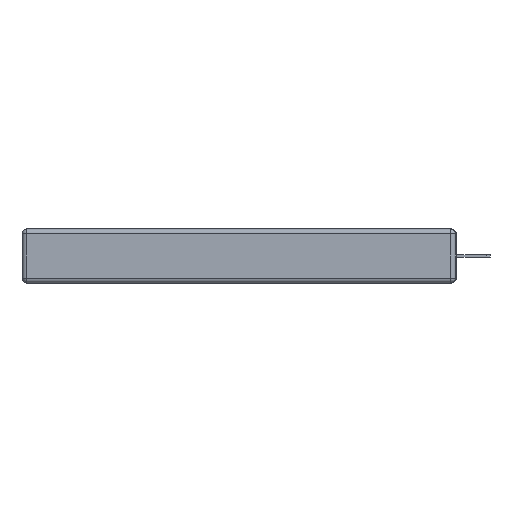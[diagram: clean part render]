
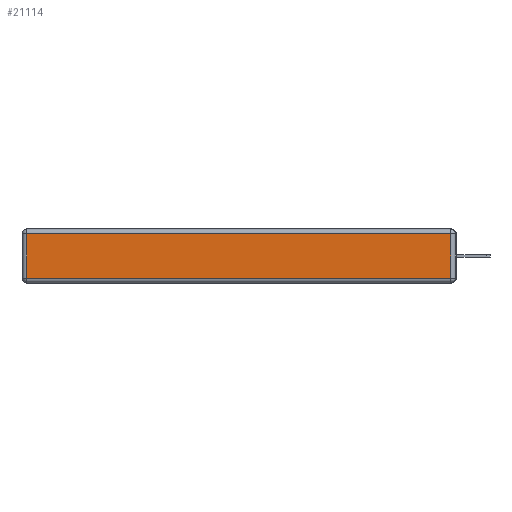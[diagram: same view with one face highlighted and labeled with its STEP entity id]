
A CAD part, left-side view. The second image highlights one B-rep face of the part: STEP entity #21114.
In plain terms, the highlighted planar face has unit normal (-1, 0, 0).
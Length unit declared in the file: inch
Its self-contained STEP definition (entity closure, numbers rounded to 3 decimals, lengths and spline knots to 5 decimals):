
#249 = ORIENTED_EDGE ( 'NONE', *, *, #13192, .T. ) ;
#598 = CARTESIAN_POINT ( 'NONE',  ( 0., 0.03, -0.03 ) ) ;
#813 = VERTEX_POINT ( 'NONE', #15859 ) ;
#1309 = DIRECTION ( 'NONE',  ( 0., 0., 1. ) ) ;
#1898 = ORIENTED_EDGE ( 'NONE', *, *, #19067, .T. ) ;
#2978 = CARTESIAN_POINT ( 'NONE',  ( 0., 0., -0.343 ) ) ;
#3934 = EDGE_LOOP ( 'NONE', ( #6004, #249, #11787, #1898 ) ) ;
#4666 = VECTOR ( 'NONE', #4872, 39.37008 ) ;
#4684 = DIRECTION ( 'NONE',  ( 0., 0., -1. ) ) ;
#4872 = DIRECTION ( 'NONE',  ( 0., 0., 1. ) ) ;
#5842 = VERTEX_POINT ( 'NONE', #19207 ) ;
#6004 = ORIENTED_EDGE ( 'NONE', *, *, #18140, .T. ) ;
#6305 = PLANE ( 'NONE',  #6589 ) ;
#6589 = AXIS2_PLACEMENT_3D ( 'NONE', #2978, #16469, #1309 ) ;
#7566 = CARTESIAN_POINT ( 'NONE',  ( 0., 0., -0.313 ) ) ;
#10645 = DIRECTION ( 'NONE',  ( 0., -1., 0. ) ) ;
#10928 = EDGE_CURVE ( 'NONE', #14163, #813, #13548, .T. ) ;
#11065 = VERTEX_POINT ( 'NONE', #17620 ) ;
#11787 = ORIENTED_EDGE ( 'NONE', *, *, #10928, .T. ) ;
#12101 = CARTESIAN_POINT ( 'NONE',  ( 0., 2.75, -0.03 ) ) ;
#13192 = EDGE_CURVE ( 'NONE', #11065, #14163, #13281, .T. ) ;
#13281 = LINE ( 'NONE', #20012, #4666 ) ;
#13548 = LINE ( 'NONE', #12101, #15796 ) ;
#14099 = LINE ( 'NONE', #7566, #18890 ) ;
#14163 = VERTEX_POINT ( 'NONE', #598 ) ;
#14623 = VECTOR ( 'NONE', #4684, 39.37008 ) ;
#15796 = VECTOR ( 'NONE', #18829, 39.37008 ) ;
#15859 = CARTESIAN_POINT ( 'NONE',  ( 0., 2.72, -0.03 ) ) ;
#16148 = FACE_OUTER_BOUND ( 'NONE', #3934, .T. ) ;
#16469 = DIRECTION ( 'NONE',  ( -1., 0., 0. ) ) ;
#17620 = CARTESIAN_POINT ( 'NONE',  ( 0., 0.03, -0.313 ) ) ;
#18140 = EDGE_CURVE ( 'NONE', #5842, #11065, #14099, .T. ) ;
#18829 = DIRECTION ( 'NONE',  ( 0., 1., 0. ) ) ;
#18890 = VECTOR ( 'NONE', #10645, 39.37008 ) ;
#19067 = EDGE_CURVE ( 'NONE', #813, #5842, #19617, .T. ) ;
#19207 = CARTESIAN_POINT ( 'NONE',  ( 0., 2.72, -0.313 ) ) ;
#19617 = LINE ( 'NONE', #19829, #14623 ) ;
#19829 = CARTESIAN_POINT ( 'NONE',  ( 0., 2.72, -0.343 ) ) ;
#20012 = CARTESIAN_POINT ( 'NONE',  ( 0., 0.03, -0.343 ) ) ;
#21114 = ADVANCED_FACE ( 'NONE', ( #16148 ), #6305, .T. ) ;
